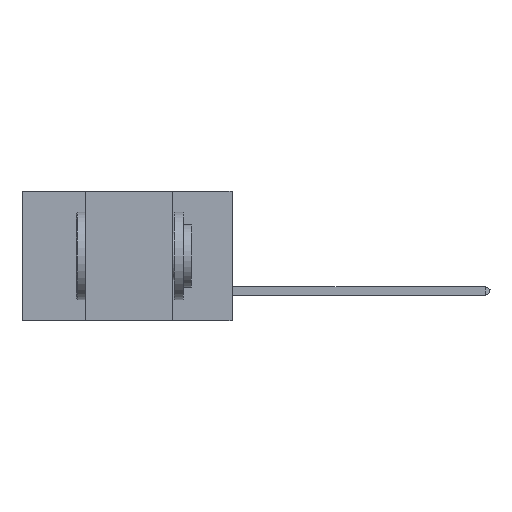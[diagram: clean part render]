
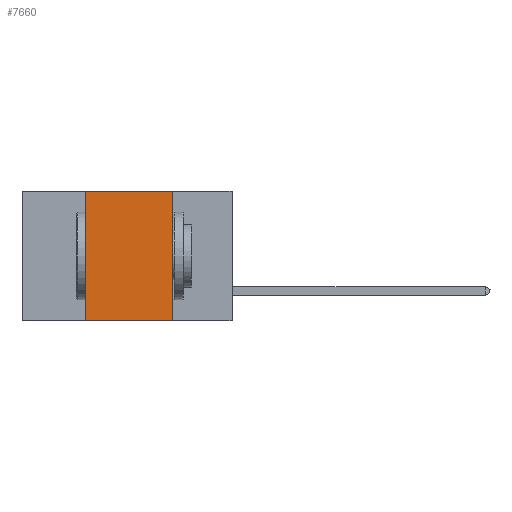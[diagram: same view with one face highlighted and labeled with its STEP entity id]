
A CAD part, left-side view. The second image highlights one B-rep face of the part: STEP entity #7660.
In plain terms, the highlighted planar face has unit normal (-1, 0, 0).
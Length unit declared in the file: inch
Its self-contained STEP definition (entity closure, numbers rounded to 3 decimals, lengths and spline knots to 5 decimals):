
#785 = EDGE_LOOP ( 'NONE', ( #8836, #3545, #7659, #4436 ) ) ;
#828 = CARTESIAN_POINT ( 'NONE',  ( 0., 0.17, 0. ) ) ;
#931 = VERTEX_POINT ( 'NONE', #828 ) ;
#1812 = EDGE_CURVE ( 'NONE', #931, #9095, #9056, .T. ) ;
#1923 = DIRECTION ( 'NONE',  ( 0., 0., 1. ) ) ;
#2002 = CARTESIAN_POINT ( 'NONE',  ( 0., 0.42, 0. ) ) ;
#2661 = CARTESIAN_POINT ( 'NONE',  ( 0., 0.6, -0.37 ) ) ;
#3132 = VECTOR ( 'NONE', #5772, 39.37008 ) ;
#3455 = CARTESIAN_POINT ( 'NONE',  ( 0., 0.17, -0.37 ) ) ;
#3470 = LINE ( 'NONE', #2002, #5773 ) ;
#3545 = ORIENTED_EDGE ( 'NONE', *, *, #6711, .F. ) ;
#3570 = CARTESIAN_POINT ( 'NONE',  ( 0., 0.42, 0. ) ) ;
#3728 = DIRECTION ( 'NONE',  ( 0., 0., -1. ) ) ;
#3946 = VECTOR ( 'NONE', #3728, 39.37008 ) ;
#4297 = EDGE_CURVE ( 'NONE', #9667, #9095, #7085, .T. ) ;
#4436 = ORIENTED_EDGE ( 'NONE', *, *, #4297, .T. ) ;
#4549 = CARTESIAN_POINT ( 'NONE',  ( 0., 0.17, 0. ) ) ;
#5139 = CARTESIAN_POINT ( 'NONE',  ( 0., 0.42, -0.37 ) ) ;
#5602 = VERTEX_POINT ( 'NONE', #3570 ) ;
#5772 = DIRECTION ( 'NONE',  ( 0., -1., 0. ) ) ;
#5773 = VECTOR ( 'NONE', #1923, 39.37008 ) ;
#6017 = EDGE_CURVE ( 'NONE', #9667, #5602, #3470, .T. ) ;
#6038 = CARTESIAN_POINT ( 'NONE',  ( 0., 0.6, 0. ) ) ;
#6670 = AXIS2_PLACEMENT_3D ( 'NONE', #6038, #7600, #7563 ) ;
#6711 = EDGE_CURVE ( 'NONE', #5602, #931, #8948, .T. ) ;
#7085 = LINE ( 'NONE', #2661, #3132 ) ;
#7563 = DIRECTION ( 'NONE',  ( 0., 0., -1. ) ) ;
#7600 = DIRECTION ( 'NONE',  ( 1., 0., 0. ) ) ;
#7659 = ORIENTED_EDGE ( 'NONE', *, *, #6017, .F. ) ;
#7660 = ADVANCED_FACE ( 'NONE', ( #9958 ), #8396, .F. ) ;
#8396 = PLANE ( 'NONE',  #6670 ) ;
#8836 = ORIENTED_EDGE ( 'NONE', *, *, #1812, .F. ) ;
#8874 = DIRECTION ( 'NONE',  ( 0., -1., 0. ) ) ;
#8908 = CARTESIAN_POINT ( 'NONE',  ( 0., 0.6, 0. ) ) ;
#8948 = LINE ( 'NONE', #8908, #9848 ) ;
#9056 = LINE ( 'NONE', #4549, #3946 ) ;
#9095 = VERTEX_POINT ( 'NONE', #3455 ) ;
#9667 = VERTEX_POINT ( 'NONE', #5139 ) ;
#9848 = VECTOR ( 'NONE', #8874, 39.37008 ) ;
#9958 = FACE_OUTER_BOUND ( 'NONE', #785, .T. ) ;
